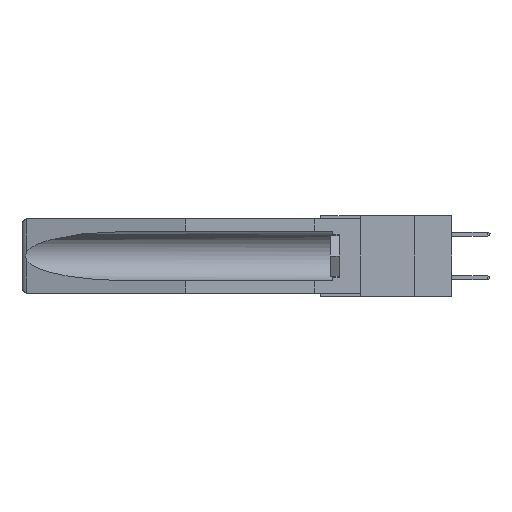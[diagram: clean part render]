
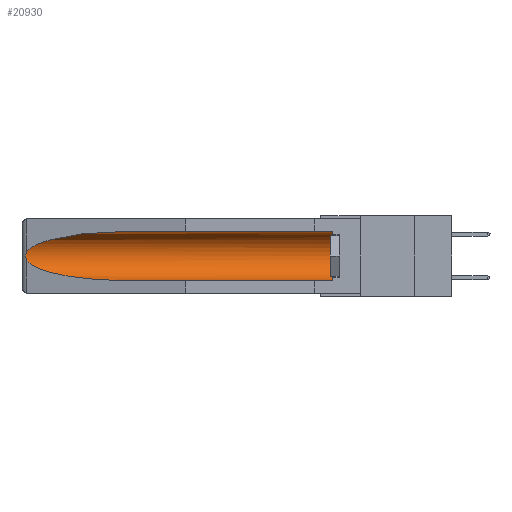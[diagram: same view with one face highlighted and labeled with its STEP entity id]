
A CAD part, left-side view. The second image highlights one B-rep face of the part: STEP entity #20930.
In plain terms, the highlighted cylindrical face has radius 2.857 mm (diameter 5.715 mm), a partial arc.
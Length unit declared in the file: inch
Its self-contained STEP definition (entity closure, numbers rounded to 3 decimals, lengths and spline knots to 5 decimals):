
#516 = CARTESIAN_POINT ( 'NONE',  ( 0.26537, 1.52718, -0.14972 ) ) ;
#768 = CARTESIAN_POINT ( 'NONE',  ( 0.155, 0.126, -0.1715 ) ) ;
#887 = CARTESIAN_POINT ( 'NONE',  ( 0.155, 1.07973, -0.059 ) ) ;
#1325 = CARTESIAN_POINT ( 'NONE',  ( 0.26597, 1.52961, -0.15275 ) ) ;
#1551 = CARTESIAN_POINT ( 'NONE',  ( 0.26597, 1.5296, -0.19026 ) ) ;
#1828 = FACE_OUTER_BOUND ( 'NONE', #1968, .T. ) ;
#1968 = EDGE_LOOP ( 'NONE', ( #19705, #18030, #27754, #8549, #3633, #3374 ) ) ;
#2290 = LINE ( 'NONE', #33005, #28830 ) ;
#2833 = AXIS2_PLACEMENT_3D ( 'NONE', #26175, #31145, #15594 ) ;
#3241 = EDGE_CURVE ( 'NONE', #22020, #24302, #9715, .T. ) ;
#3374 = ORIENTED_EDGE ( 'NONE', *, *, #9813, .T. ) ;
#3633 = ORIENTED_EDGE ( 'NONE', *, *, #18106, .T. ) ;
#4112 =( BOUNDED_CURVE ( )  B_SPLINE_CURVE ( 3, ( #23873, #26464, #21146, #23772 ),
 .UNSPECIFIED., .F., .F. ) 
 B_SPLINE_CURVE_WITH_KNOTS ( ( 4, 4 ),
 ( 0.1948, 1.5708 ),
 .UNSPECIFIED. ) 
 CURVE ( )  GEOMETRIC_REPRESENTATION_ITEM ( )  RATIONAL_B_SPLINE_CURVE ( ( 1., 0.848, 0.848, 1. ) ) 
 REPRESENTATION_ITEM ( '' )  );
#6333 = CARTESIAN_POINT ( 'NONE',  ( 0.26654, 1.53092, -0.15636 ) ) ;
#6563 = CARTESIAN_POINT ( 'NONE',  ( 0.2675, 1.53308, -0.16763 ) ) ;
#7927 = CARTESIAN_POINT ( 'NONE',  ( 0.155, 0.126, -0.059 ) ) ;
#8014 = VERTEX_POINT ( 'NONE', #19571 ) ;
#8386 = CARTESIAN_POINT ( 'NONE',  ( 0.155, 1.07973, -0.059 ) ) ;
#8549 = ORIENTED_EDGE ( 'NONE', *, *, #19470, .F. ) ;
#8808 = DIRECTION ( 'NONE',  ( 0., 1., 0. ) ) ;
#9174 = CARTESIAN_POINT ( 'NONE',  ( 0.26655, 1.53094, -0.18657 ) ) ;
#9715 = B_SPLINE_CURVE_WITH_KNOTS ( 'NONE', 3,
 ( #24720, #1325, #6333, #21936, #6563, #21702, #24614, #9174, #1551, #19544 ),
 .UNSPECIFIED., .F., .F.,
 ( 4, 2, 2, 2, 4 ),
 ( 0., 0.00029, 0.00058, 0.00087, 0.00117 ),
 .UNSPECIFIED. ) ;
#9813 = EDGE_CURVE ( 'NONE', #25687, #25106, #2290, .T. ) ;
#12139 = EDGE_CURVE ( 'NONE', #25106, #22020, #13586, .T. ) ;
#13586 =( BOUNDED_CURVE ( )  B_SPLINE_CURVE ( 3, ( #8386, #31467, #23685, #516 ),
 .UNSPECIFIED., .F., .F. ) 
 B_SPLINE_CURVE_WITH_KNOTS ( ( 4, 4 ),
 ( 4.71239, 6.08839 ),
 .UNSPECIFIED. ) 
 CURVE ( )  GEOMETRIC_REPRESENTATION_ITEM ( )  RATIONAL_B_SPLINE_CURVE ( ( 1., 0.848, 0.848, 1. ) ) 
 REPRESENTATION_ITEM ( '' )  );
#14468 = DIRECTION ( 'NONE',  ( 0., 1., 0. ) ) ;
#15594 = DIRECTION ( 'NONE',  ( 0., 0., 1. ) ) ;
#18030 = ORIENTED_EDGE ( 'NONE', *, *, #3241, .T. ) ;
#18106 = EDGE_CURVE ( 'NONE', #8014, #25687, #30004, .T. ) ;
#18724 = CARTESIAN_POINT ( 'NONE',  ( 0.26537, 1.52718, -0.19328 ) ) ;
#19470 = EDGE_CURVE ( 'NONE', #8014, #26861, #29703, .T. ) ;
#19544 = CARTESIAN_POINT ( 'NONE',  ( 0.26537, 1.52718, -0.19328 ) ) ;
#19571 = CARTESIAN_POINT ( 'NONE',  ( 0.155, 0.126, -0.284 ) ) ;
#19705 = ORIENTED_EDGE ( 'NONE', *, *, #12139, .T. ) ;
#20660 = CARTESIAN_POINT ( 'NONE',  ( 0.155, 1.07973, -0.284 ) ) ;
#20930 = ADVANCED_FACE ( 'NONE', ( #1828 ), #22722, .F. ) ;
#21146 = CARTESIAN_POINT ( 'NONE',  ( 0.21114, 1.30732, -0.284 ) ) ;
#21702 = CARTESIAN_POINT ( 'NONE',  ( 0.2675, 1.53308, -0.17534 ) ) ;
#21936 = CARTESIAN_POINT ( 'NONE',  ( 0.2673, 1.5327, -0.16383 ) ) ;
#22020 = VERTEX_POINT ( 'NONE', #27087 ) ;
#22722 = CYLINDRICAL_SURFACE ( 'NONE', #2833, 0.1125 ) ;
#23685 = CARTESIAN_POINT ( 'NONE',  ( 0.25451, 1.48313, -0.09465 ) ) ;
#23772 = CARTESIAN_POINT ( 'NONE',  ( 0.155, 1.07973, -0.284 ) ) ;
#23873 = CARTESIAN_POINT ( 'NONE',  ( 0.26537, 1.52718, -0.19328 ) ) ;
#24302 = VERTEX_POINT ( 'NONE', #18724 ) ;
#24614 = CARTESIAN_POINT ( 'NONE',  ( 0.2673, 1.53269, -0.17917 ) ) ;
#24720 = CARTESIAN_POINT ( 'NONE',  ( 0.26537, 1.52718, -0.14972 ) ) ;
#25106 = VERTEX_POINT ( 'NONE', #887 ) ;
#25687 = VERTEX_POINT ( 'NONE', #7927 ) ;
#26175 = CARTESIAN_POINT ( 'NONE',  ( 0.155, -0.30754, -0.1715 ) ) ;
#26464 = CARTESIAN_POINT ( 'NONE',  ( 0.25451, 1.48313, -0.24835 ) ) ;
#26861 = VERTEX_POINT ( 'NONE', #20660 ) ;
#27087 = CARTESIAN_POINT ( 'NONE',  ( 0.26537, 1.52718, -0.14972 ) ) ;
#27754 = ORIENTED_EDGE ( 'NONE', *, *, #33185, .T. ) ;
#28830 = VECTOR ( 'NONE', #8808, 39.37008 ) ;
#28857 = DIRECTION ( 'NONE',  ( 0., -1., 0. ) ) ;
#29703 = LINE ( 'NONE', #29928, #32917 ) ;
#29928 = CARTESIAN_POINT ( 'NONE',  ( 0.155, -0.30754, -0.284 ) ) ;
#29943 = AXIS2_PLACEMENT_3D ( 'NONE', #768, #28857, #31387 ) ;
#30004 = CIRCLE ( 'NONE', #29943, 0.1125 ) ;
#31145 = DIRECTION ( 'NONE',  ( 0., 1., 0. ) ) ;
#31387 = DIRECTION ( 'NONE',  ( 0., 0., 1. ) ) ;
#31467 = CARTESIAN_POINT ( 'NONE',  ( 0.21114, 1.30732, -0.059 ) ) ;
#32917 = VECTOR ( 'NONE', #14468, 39.37008 ) ;
#33005 = CARTESIAN_POINT ( 'NONE',  ( 0.155, -0.30754, -0.059 ) ) ;
#33185 = EDGE_CURVE ( 'NONE', #24302, #26861, #4112, .T. ) ;
